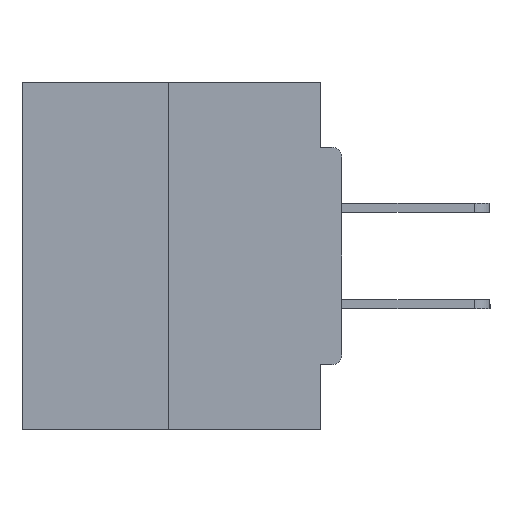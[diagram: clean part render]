
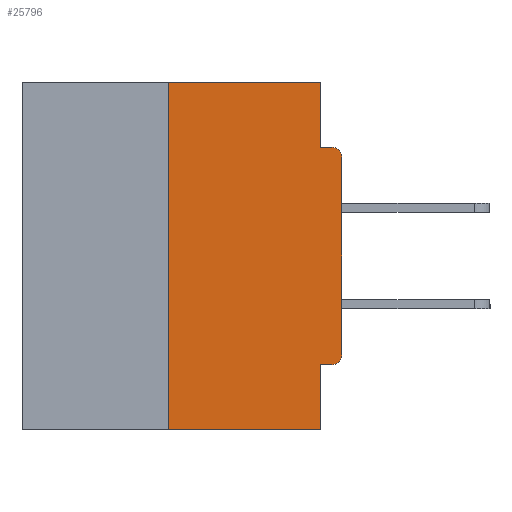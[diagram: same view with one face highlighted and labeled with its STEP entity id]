
A CAD part, left-side view. The second image highlights one B-rep face of the part: STEP entity #25796.
In plain terms, the highlighted planar face has unit normal (-1, 0, 0).
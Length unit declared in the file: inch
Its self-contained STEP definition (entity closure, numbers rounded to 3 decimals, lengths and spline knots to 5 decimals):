
#879 = DIRECTION ( 'NONE',  ( 0., 0., -1. ) ) ;
#1850 = VERTEX_POINT ( 'NONE', #40387 ) ;
#2873 = LINE ( 'NONE', #28488, #35206 ) ;
#3790 = LINE ( 'NONE', #17487, #35140 ) ;
#4006 = CARTESIAN_POINT ( 'NONE',  ( 0., 0.031, -0.5 ) ) ;
#4122 = VECTOR ( 'NONE', #22711, 39.37008 ) ;
#4284 = DIRECTION ( 'NONE',  ( 0., -1., 0. ) ) ;
#4716 = CARTESIAN_POINT ( 'NONE',  ( 0., 0.031, -0.0935 ) ) ;
#4730 = DIRECTION ( 'NONE',  ( 0., -1., 0. ) ) ;
#4861 = VERTEX_POINT ( 'NONE', #32353 ) ;
#5492 = VECTOR ( 'NONE', #4284, 39.37008 ) ;
#6745 = CARTESIAN_POINT ( 'NONE',  ( 0., 0.25, 0. ) ) ;
#6846 = ORIENTED_EDGE ( 'NONE', *, *, #29486, .F. ) ;
#7050 = VERTEX_POINT ( 'NONE', #22130 ) ;
#7848 = EDGE_CURVE ( 'NONE', #39246, #12923, #34133, .T. ) ;
#8721 = VERTEX_POINT ( 'NONE', #4006 ) ;
#8833 = CARTESIAN_POINT ( 'NONE',  ( 0., 0.015, -0.1085 ) ) ;
#8835 = VERTEX_POINT ( 'NONE', #32745 ) ;
#9888 = EDGE_CURVE ( 'NONE', #8835, #8721, #11353, .T. ) ;
#10048 = AXIS2_PLACEMENT_3D ( 'NONE', #8833, #30760, #39674 ) ;
#11255 = EDGE_CURVE ( 'NONE', #4861, #8721, #25050, .T. ) ;
#11353 = LINE ( 'NONE', #29744, #5492 ) ;
#12923 = VERTEX_POINT ( 'NONE', #39758 ) ;
#13111 = ORIENTED_EDGE ( 'NONE', *, *, #9888, .T. ) ;
#13286 = DIRECTION ( 'NONE',  ( 0., 0., 1. ) ) ;
#13379 = VECTOR ( 'NONE', #29527, 39.37008 ) ;
#14096 = VERTEX_POINT ( 'NONE', #30002 ) ;
#14872 = DIRECTION ( 'NONE',  ( 0., 0., -1. ) ) ;
#15392 = CARTESIAN_POINT ( 'NONE',  ( 0., 0., 0. ) ) ;
#15463 = ORIENTED_EDGE ( 'NONE', *, *, #7848, .T. ) ;
#16142 = EDGE_CURVE ( 'NONE', #7050, #25917, #25732, .T. ) ;
#16812 = CARTESIAN_POINT ( 'NONE',  ( 0., 0., -0.4065 ) ) ;
#16973 = CARTESIAN_POINT ( 'NONE',  ( 0., 0.25, 0. ) ) ;
#17088 = EDGE_CURVE ( 'NONE', #1850, #39246, #22755, .T. ) ;
#17487 = CARTESIAN_POINT ( 'NONE',  ( 0., 0., -0.0935 ) ) ;
#18422 = DIRECTION ( 'NONE',  ( 0., 0., 1. ) ) ;
#18466 = LINE ( 'NONE', #6745, #34129 ) ;
#19554 = CARTESIAN_POINT ( 'NONE',  ( 0., 0.031, 0. ) ) ;
#19728 = ORIENTED_EDGE ( 'NONE', *, *, #17088, .T. ) ;
#21770 = VECTOR ( 'NONE', #18422, 39.37008 ) ;
#22130 = CARTESIAN_POINT ( 'NONE',  ( 0., 0.031, 0. ) ) ;
#22375 = DIRECTION ( 'NONE',  ( 0., -1., 0. ) ) ;
#22549 = EDGE_CURVE ( 'NONE', #14096, #1850, #26054, .T. ) ;
#22711 = DIRECTION ( 'NONE',  ( 0., 0., -1. ) ) ;
#22755 = LINE ( 'NONE', #15392, #21770 ) ;
#22816 = ORIENTED_EDGE ( 'NONE', *, *, #32123, .F. ) ;
#23076 = VECTOR ( 'NONE', #14872, 39.37008 ) ;
#23390 = FACE_OUTER_BOUND ( 'NONE', #25799, .T. ) ;
#23517 = ORIENTED_EDGE ( 'NONE', *, *, #35403, .F. ) ;
#25050 = LINE ( 'NONE', #39786, #23076 ) ;
#25723 = ORIENTED_EDGE ( 'NONE', *, *, #16142, .F. ) ;
#25732 = LINE ( 'NONE', #19554, #4122 ) ;
#25796 = ADVANCED_FACE ( 'NONE', ( #23390 ), #35150, .F. ) ;
#25799 = EDGE_LOOP ( 'NONE', ( #23517, #32953, #13111, #36771, #22816, #33943, #19728, #15463, #6846, #25723 ) ) ;
#25917 = VERTEX_POINT ( 'NONE', #4716 ) ;
#26054 = CIRCLE ( 'NONE', #38729, 0.015 ) ;
#26123 = EDGE_CURVE ( 'NONE', #8835, #33334, #18466, .T. ) ;
#28488 = CARTESIAN_POINT ( 'NONE',  ( 0., 0.46, 0. ) ) ;
#29227 = DIRECTION ( 'NONE',  ( 1., 0., 0. ) ) ;
#29486 = EDGE_CURVE ( 'NONE', #25917, #12923, #3790, .T. ) ;
#29527 = DIRECTION ( 'NONE',  ( 0., 1., 0. ) ) ;
#29723 = AXIS2_PLACEMENT_3D ( 'NONE', #35274, #29227, #879 ) ;
#29744 = CARTESIAN_POINT ( 'NONE',  ( 0., 0.46, -0.5 ) ) ;
#30002 = CARTESIAN_POINT ( 'NONE',  ( 0., 0.015, -0.4065 ) ) ;
#30760 = DIRECTION ( 'NONE',  ( -1., 0., 0. ) ) ;
#31411 = DIRECTION ( 'NONE',  ( 0., 0., -1. ) ) ;
#31512 = LINE ( 'NONE', #16812, #13379 ) ;
#32123 = EDGE_CURVE ( 'NONE', #14096, #4861, #31512, .T. ) ;
#32353 = CARTESIAN_POINT ( 'NONE',  ( 0., 0.031, -0.4065 ) ) ;
#32745 = CARTESIAN_POINT ( 'NONE',  ( 0., 0.25, -0.5 ) ) ;
#32953 = ORIENTED_EDGE ( 'NONE', *, *, #26123, .F. ) ;
#33334 = VERTEX_POINT ( 'NONE', #16973 ) ;
#33943 = ORIENTED_EDGE ( 'NONE', *, *, #22549, .T. ) ;
#34129 = VECTOR ( 'NONE', #13286, 39.37008 ) ;
#34133 = CIRCLE ( 'NONE', #10048, 0.015 ) ;
#35140 = VECTOR ( 'NONE', #4730, 39.37008 ) ;
#35150 = PLANE ( 'NONE',  #29723 ) ;
#35206 = VECTOR ( 'NONE', #22375, 39.37008 ) ;
#35274 = CARTESIAN_POINT ( 'NONE',  ( 0., 0.46, 0. ) ) ;
#35403 = EDGE_CURVE ( 'NONE', #33334, #7050, #2873, .T. ) ;
#36771 = ORIENTED_EDGE ( 'NONE', *, *, #11255, .F. ) ;
#37554 = CARTESIAN_POINT ( 'NONE',  ( 0., 0., -0.1085 ) ) ;
#37867 = DIRECTION ( 'NONE',  ( -1., 0., 0. ) ) ;
#38729 = AXIS2_PLACEMENT_3D ( 'NONE', #40443, #37867, #31411 ) ;
#39246 = VERTEX_POINT ( 'NONE', #37554 ) ;
#39674 = DIRECTION ( 'NONE',  ( 0., 0., -1. ) ) ;
#39758 = CARTESIAN_POINT ( 'NONE',  ( 0., 0.015, -0.0935 ) ) ;
#39786 = CARTESIAN_POINT ( 'NONE',  ( 0., 0.031, -0.5 ) ) ;
#40387 = CARTESIAN_POINT ( 'NONE',  ( 0., 0., -0.3915 ) ) ;
#40443 = CARTESIAN_POINT ( 'NONE',  ( 0., 0.015, -0.3915 ) ) ;
